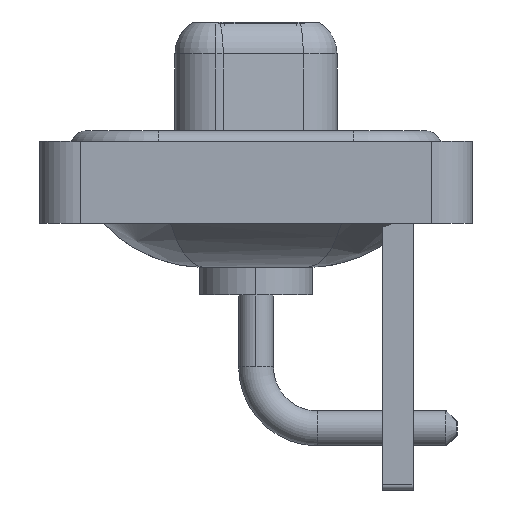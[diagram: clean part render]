
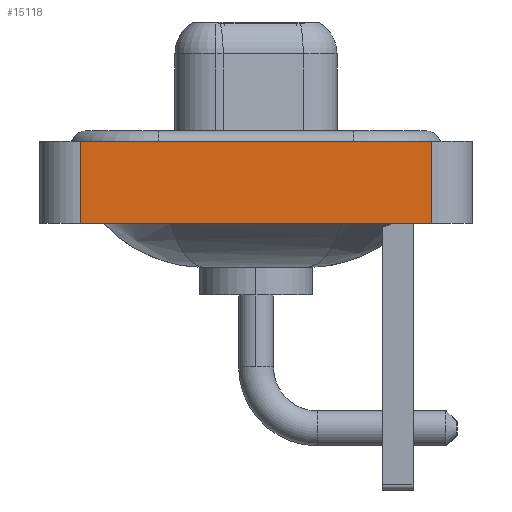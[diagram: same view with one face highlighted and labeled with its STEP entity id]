
A CAD part, left-side view. The second image highlights one B-rep face of the part: STEP entity #15118.
In plain terms, the highlighted planar face has unit normal (-1, 0, 0).
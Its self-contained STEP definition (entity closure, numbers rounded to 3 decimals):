
#1422 = PLANE ( 'NONE',  #11692 ) ;
#1655 = DIRECTION ( 'NONE',  ( 0., -1., 0. ) ) ;
#1770 = DIRECTION ( 'NONE',  ( 0., 0., 1. ) ) ;
#1956 = LINE ( 'NONE', #7415, #4751 ) ;
#2259 = FACE_OUTER_BOUND ( 'NONE', #4433, .T. ) ;
#2510 = ORIENTED_EDGE ( 'NONE', *, *, #3261, .F. ) ;
#3068 = VECTOR ( 'NONE', #3471, 1000. ) ;
#3261 = EDGE_CURVE ( 'NONE', #11112, #8724, #1956, .T. ) ;
#3471 = DIRECTION ( 'NONE',  ( 0., -1., 0. ) ) ;
#3571 = CARTESIAN_POINT ( 'NONE',  ( -7.3, -8.55, -3.6 ) ) ;
#3792 = CARTESIAN_POINT ( 'NONE',  ( -7.3, 8.55, 0.4 ) ) ;
#4216 = DIRECTION ( 'NONE',  ( 0., 0., 1. ) ) ;
#4390 = LINE ( 'NONE', #4483, #18133 ) ;
#4433 = EDGE_LOOP ( 'NONE', ( #7716, #16744, #2510, #4658 ) ) ;
#4483 = CARTESIAN_POINT ( 'NONE',  ( -7.3, -8.55, -3.6 ) ) ;
#4658 = ORIENTED_EDGE ( 'NONE', *, *, #13289, .T. ) ;
#4751 = VECTOR ( 'NONE', #1770, 1000. ) ;
#4951 = CARTESIAN_POINT ( 'NONE',  ( -7.3, -8.55, -3.6 ) ) ;
#5396 = DIRECTION ( 'NONE',  ( -1., 0., 0. ) ) ;
#7380 = VERTEX_POINT ( 'NONE', #7523 ) ;
#7394 = LINE ( 'NONE', #13024, #11922 ) ;
#7415 = CARTESIAN_POINT ( 'NONE',  ( -7.3, 8.55, -3.6 ) ) ;
#7523 = CARTESIAN_POINT ( 'NONE',  ( -7.3, -8.55, 0.4 ) ) ;
#7716 = ORIENTED_EDGE ( 'NONE', *, *, #16513, .T. ) ;
#8724 = VERTEX_POINT ( 'NONE', #3792 ) ;
#11112 = VERTEX_POINT ( 'NONE', #17772 ) ;
#11692 = AXIS2_PLACEMENT_3D ( 'NONE', #13899, #5396, #12340 ) ;
#11922 = VECTOR ( 'NONE', #1655, 1000. ) ;
#12172 = LINE ( 'NONE', #4951, #3068 ) ;
#12340 = DIRECTION ( 'NONE',  ( 0., 0., 1. ) ) ;
#13024 = CARTESIAN_POINT ( 'NONE',  ( -7.3, -8.55, 0.4 ) ) ;
#13289 = EDGE_CURVE ( 'NONE', #11112, #14584, #12172, .T. ) ;
#13899 = CARTESIAN_POINT ( 'NONE',  ( -7.3, -8.55, -3.6 ) ) ;
#14584 = VERTEX_POINT ( 'NONE', #3571 ) ;
#15118 = ADVANCED_FACE ( 'NONE', ( #2259 ), #1422, .T. ) ;
#16513 = EDGE_CURVE ( 'NONE', #14584, #7380, #4390, .T. ) ;
#16744 = ORIENTED_EDGE ( 'NONE', *, *, #17474, .F. ) ;
#17474 = EDGE_CURVE ( 'NONE', #8724, #7380, #7394, .T. ) ;
#17772 = CARTESIAN_POINT ( 'NONE',  ( -7.3, 8.55, -3.6 ) ) ;
#18133 = VECTOR ( 'NONE', #4216, 1000. ) ;
